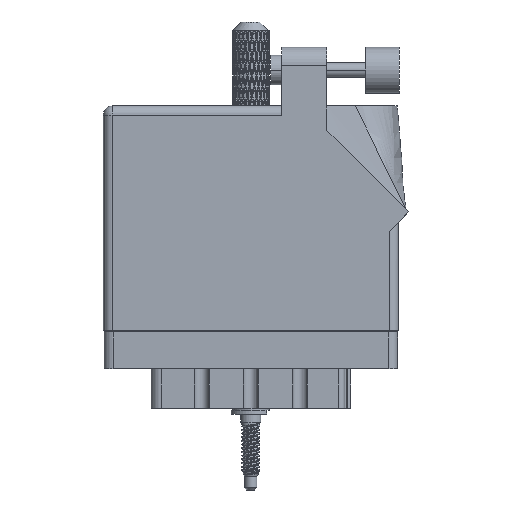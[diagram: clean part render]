
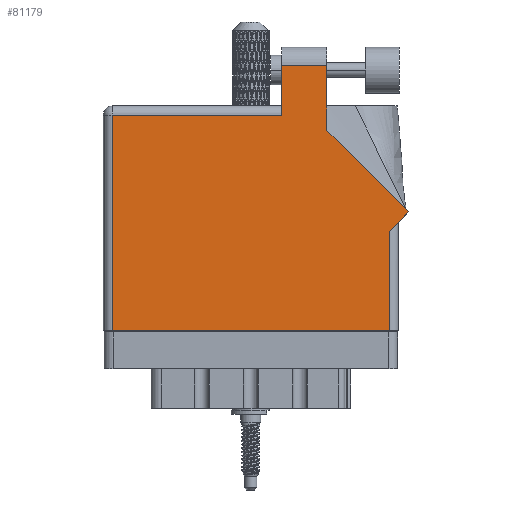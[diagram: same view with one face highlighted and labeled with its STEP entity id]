
A CAD part, front view. The second image highlights one B-rep face of the part: STEP entity #81179.
In plain terms, the highlighted face is planar.
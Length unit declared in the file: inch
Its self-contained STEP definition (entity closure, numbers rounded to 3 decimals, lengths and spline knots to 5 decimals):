
#4209 = EDGE_LOOP ( 'NONE', ( #34952, #86333, #71186, #10132, #7238, #51080, #5123, #5559, #33876 ) ) ;
#5123 = ORIENTED_EDGE ( 'NONE', *, *, #42403, .T. ) ;
#5559 = ORIENTED_EDGE ( 'NONE', *, *, #55200, .T. ) ;
#7238 = ORIENTED_EDGE ( 'NONE', *, *, #67846, .T. ) ;
#9123 = VERTEX_POINT ( 'NONE', #22641 ) ;
#10132 = ORIENTED_EDGE ( 'NONE', *, *, #55882, .T. ) ;
#11151 = CARTESIAN_POINT ( 'NONE',  ( 1.948, 0., 0. ) ) ;
#14968 = VECTOR ( 'NONE', #72763, 39.37008 ) ;
#16213 = DIRECTION ( 'NONE',  ( -1., 0., 0. ) ) ;
#16458 = VERTEX_POINT ( 'NONE', #36976 ) ;
#19156 = LINE ( 'NONE', #44349, #29545 ) ;
#19865 = DIRECTION ( 'NONE',  ( -0.707, 0.707, 0. ) ) ;
#22359 = CARTESIAN_POINT ( 'NONE',  ( 0.062, 0., 0. ) ) ;
#22641 = CARTESIAN_POINT ( 'NONE',  ( 1.524, 1.805, 0. ) ) ;
#23733 = CARTESIAN_POINT ( 'NONE',  ( 1.217, 1.805, 0. ) ) ;
#26973 = VECTOR ( 'NONE', #19865, 39.37008 ) ;
#27599 = EDGE_CURVE ( 'NONE', #102342, #93800, #19156, .T. ) ;
#29545 = VECTOR ( 'NONE', #43991, 39.37008 ) ;
#32219 = LINE ( 'NONE', #69885, #68111 ) ;
#33876 = ORIENTED_EDGE ( 'NONE', *, *, #103506, .T. ) ;
#34952 = ORIENTED_EDGE ( 'NONE', *, *, #86882, .T. ) ;
#36976 = CARTESIAN_POINT ( 'NONE',  ( 1.217, 1.468, 0. ) ) ;
#37305 = CARTESIAN_POINT ( 'NONE',  ( 0.062, 0., 0. ) ) ;
#42403 = EDGE_CURVE ( 'NONE', #93800, #85074, #32219, .T. ) ;
#43991 = DIRECTION ( 'NONE',  ( 1., 0., 0. ) ) ;
#44092 = DIRECTION ( 'NONE',  ( 0., -1., 0. ) ) ;
#44349 = CARTESIAN_POINT ( 'NONE',  ( 0., 0., 0. ) ) ;
#47227 = VERTEX_POINT ( 'NONE', #65233 ) ;
#47598 = DIRECTION ( 'NONE',  ( 0., 0., -1. ) ) ;
#48313 = CARTESIAN_POINT ( 'NONE',  ( 0., 1.53, 0. ) ) ;
#51080 = ORIENTED_EDGE ( 'NONE', *, *, #27599, .T. ) ;
#54215 = CARTESIAN_POINT ( 'NONE',  ( 1.524, 1.36442, 0. ) ) ;
#54621 = CARTESIAN_POINT ( 'NONE',  ( 1.524, 1.36442, 0. ) ) ;
#55200 = EDGE_CURVE ( 'NONE', #85074, #102037, #82759, .T. ) ;
#55781 = CARTESIAN_POINT ( 'NONE',  ( 2.01, 0.737, 0. ) ) ;
#55882 = EDGE_CURVE ( 'NONE', #16458, #47227, #59544, .T. ) ;
#58759 = LINE ( 'NONE', #92287, #14968 ) ;
#59544 = LINE ( 'NONE', #92615, #100873 ) ;
#60096 = DIRECTION ( 'NONE',  ( 0., -1., 0. ) ) ;
#63926 = LINE ( 'NONE', #54621, #105322 ) ;
#64120 = DIRECTION ( 'NONE',  ( 0., 1., 0. ) ) ;
#65212 = LINE ( 'NONE', #37305, #80719 ) ;
#65233 = CARTESIAN_POINT ( 'NONE',  ( 0.062, 1.468, 0. ) ) ;
#67846 = EDGE_CURVE ( 'NONE', #47227, #102342, #65212, .T. ) ;
#68111 = VECTOR ( 'NONE', #64120, 39.37008 ) ;
#68293 = CARTESIAN_POINT ( 'NONE',  ( 1.217, 1.53, 0. ) ) ;
#69446 = VERTEX_POINT ( 'NONE', #23733 ) ;
#69885 = CARTESIAN_POINT ( 'NONE',  ( 1.948, 0.737, 0. ) ) ;
#70683 = CARTESIAN_POINT ( 'NONE',  ( 2.08071, 0.80771, 0. ) ) ;
#71186 = ORIENTED_EDGE ( 'NONE', *, *, #80026, .T. ) ;
#72371 = PLANE ( 'NONE',  #90917 ) ;
#72398 = VERTEX_POINT ( 'NONE', #54215 ) ;
#72763 = DIRECTION ( 'NONE',  ( -1., 0., 0. ) ) ;
#74810 = CARTESIAN_POINT ( 'NONE',  ( 1.948, 0.675, 0. ) ) ;
#78126 = CARTESIAN_POINT ( 'NONE',  ( 2.08071, 0.80771, 0. ) ) ;
#79720 = LINE ( 'NONE', #78126, #26973 ) ;
#80026 = EDGE_CURVE ( 'NONE', #69446, #16458, #92628, .T. ) ;
#80453 = DIRECTION ( 'NONE',  ( 0., 1., 0. ) ) ;
#80719 = VECTOR ( 'NONE', #44092, 39.37008 ) ;
#81179 = ADVANCED_FACE ( 'NONE', ( #89812 ), #72371, .F. ) ;
#82759 = LINE ( 'NONE', #55781, #102230 ) ;
#85074 = VERTEX_POINT ( 'NONE', #74810 ) ;
#86333 = ORIENTED_EDGE ( 'NONE', *, *, #106092, .T. ) ;
#86882 = EDGE_CURVE ( 'NONE', #72398, #9123, #63926, .T. ) ;
#89812 = FACE_OUTER_BOUND ( 'NONE', #4209, .T. ) ;
#90917 = AXIS2_PLACEMENT_3D ( 'NONE', #48313, #47598, #16213 ) ;
#92287 = CARTESIAN_POINT ( 'NONE',  ( 1.217, 1.805, 0. ) ) ;
#92615 = CARTESIAN_POINT ( 'NONE',  ( 0., 1.468, 0. ) ) ;
#92628 = LINE ( 'NONE', #68293, #104320 ) ;
#93800 = VERTEX_POINT ( 'NONE', #11151 ) ;
#95885 = DIRECTION ( 'NONE',  ( 0.707, 0.707, 0. ) ) ;
#100873 = VECTOR ( 'NONE', #100964, 39.37008 ) ;
#100964 = DIRECTION ( 'NONE',  ( -1., 0., 0. ) ) ;
#102037 = VERTEX_POINT ( 'NONE', #70683 ) ;
#102230 = VECTOR ( 'NONE', #95885, 39.37008 ) ;
#102342 = VERTEX_POINT ( 'NONE', #22359 ) ;
#103506 = EDGE_CURVE ( 'NONE', #102037, #72398, #79720, .T. ) ;
#104320 = VECTOR ( 'NONE', #60096, 39.37008 ) ;
#105322 = VECTOR ( 'NONE', #80453, 39.37008 ) ;
#106092 = EDGE_CURVE ( 'NONE', #9123, #69446, #58759, .T. ) ;
